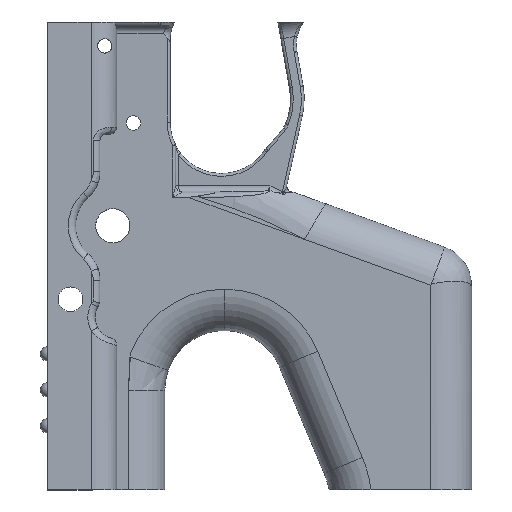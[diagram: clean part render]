
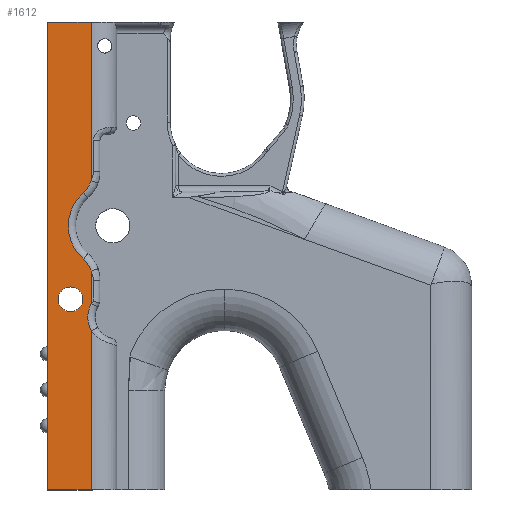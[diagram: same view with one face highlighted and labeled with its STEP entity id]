
A CAD part, left-side view. The second image highlights one B-rep face of the part: STEP entity #1612.
In plain terms, the highlighted planar face has unit normal (-1, 0, 0).
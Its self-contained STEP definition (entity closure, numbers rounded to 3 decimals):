
#29 = ORIENTED_EDGE ( 'NONE', *, *, #5917, .T. ) ;
#49 = ORIENTED_EDGE ( 'NONE', *, *, #7983, .F. ) ;
#68 = VERTEX_POINT ( 'NONE', #8819 ) ;
#126 = CARTESIAN_POINT ( 'NONE',  ( 4.253, 39.359, 4.07 ) ) ;
#310 = CARTESIAN_POINT ( 'NONE',  ( 4.253, 33.602, -8.151 ) ) ;
#328 = ORIENTED_EDGE ( 'NONE', *, *, #7733, .F. ) ;
#339 = EDGE_CURVE ( 'NONE', #5930, #7018, #5388, .T. ) ;
#431 = EDGE_CURVE ( 'NONE', #11280, #6899, #5611, .T. ) ;
#524 = ORIENTED_EDGE ( 'NONE', *, *, #3425, .F. ) ;
#691 = AXIS2_PLACEMENT_3D ( 'NONE', #8470, #8398, #8358 ) ;
#1302 = EDGE_LOOP ( 'NONE', ( #49, #524 ) ) ;
#1612 = ADVANCED_FACE ( 'NONE', ( #8592, #8515 ), #9590, .T. ) ;
#1860 = VERTEX_POINT ( 'NONE', #7393 ) ;
#1989 = EDGE_CURVE ( 'NONE', #10378, #4350, #9671, .T. ) ;
#2120 = EDGE_LOOP ( 'NONE', ( #10586, #9983, #5983, #11621, #10898, #5056, #29, #11926, #9533, #328 ) ) ;
#2543 = CARTESIAN_POINT ( 'NONE',  ( 4.253, 33.602, -52.337 ) ) ;
#2714 = EDGE_CURVE ( 'NONE', #4350, #5930, #12246, .T. ) ;
#2930 = CARTESIAN_POINT ( 'NONE',  ( 4.253, 39.359, 0.641 ) ) ;
#3131 = CARTESIAN_POINT ( 'NONE',  ( 4.253, 45.721, -52.337 ) ) ;
#3237 = LINE ( 'NONE', #7360, #3402 ) ;
#3402 = VECTOR ( 'NONE', #7688, 1000. ) ;
#3425 = EDGE_CURVE ( 'NONE', #6304, #6214, #4890, .T. ) ;
#3901 = DIRECTION ( 'NONE',  ( 0., 0., 1. ) ) ;
#3908 = VERTEX_POINT ( 'NONE', #3131 ) ;
#3967 = AXIS2_PLACEMENT_3D ( 'NONE', #4421, #3987, #4104 ) ;
#3987 = DIRECTION ( 'NONE',  ( 1., 0., 0. ) ) ;
#4104 = DIRECTION ( 'NONE',  ( 0., 0., 1. ) ) ;
#4350 = VERTEX_POINT ( 'NONE', #310 ) ;
#4421 = CARTESIAN_POINT ( 'NONE',  ( 4.253, 26.544, -4.363 ) ) ;
#4700 = DIRECTION ( 'NONE',  ( 0., 0., 1. ) ) ;
#4721 = CARTESIAN_POINT ( 'NONE',  ( 4.253, 33.602, 8.466 ) ) ;
#4752 = DIRECTION ( 'NONE',  ( 1., 0., 0. ) ) ;
#4765 = CARTESIAN_POINT ( 'NONE',  ( 4.253, 27.586, 21.037 ) ) ;
#4802 = CARTESIAN_POINT ( 'NONE',  ( 4.253, 35.831, 30.248 ) ) ;
#4890 = CIRCLE ( 'NONE', #691, 3.429 ) ;
#5056 = ORIENTED_EDGE ( 'NONE', *, *, #431, .T. ) ;
#5057 = AXIS2_PLACEMENT_3D ( 'NONE', #11637, #11622, #11606 ) ;
#5104 = DIRECTION ( 'NONE',  ( 0., 0., 1. ) ) ;
#5123 = EDGE_CURVE ( 'NONE', #7018, #12209, #7668, .T. ) ;
#5266 = CARTESIAN_POINT ( 'NONE',  ( 4.253, 41.167, 5.866 ) ) ;
#5302 = DIRECTION ( 'NONE',  ( -1., 0., 0. ) ) ;
#5388 = LINE ( 'NONE', #9391, #5407 ) ;
#5407 = VECTOR ( 'NONE', #9187, 1000. ) ;
#5438 = EDGE_CURVE ( 'NONE', #12209, #11280, #6070, .T. ) ;
#5611 = CIRCLE ( 'NONE', #5057, 8. ) ;
#5917 = EDGE_CURVE ( 'NONE', #6899, #68, #3237, .T. ) ;
#5930 = VERTEX_POINT ( 'NONE', #7248 ) ;
#5983 = ORIENTED_EDGE ( 'NONE', *, *, #339, .T. ) ;
#6025 = DIRECTION ( 'NONE',  ( 0., 0., 1. ) ) ;
#6070 = CIRCLE ( 'NONE', #11005, 12.362 ) ;
#6175 = AXIS2_PLACEMENT_3D ( 'NONE', #5266, #5302, #5104 ) ;
#6214 = VERTEX_POINT ( 'NONE', #126 ) ;
#6304 = VERTEX_POINT ( 'NONE', #10515 ) ;
#6432 = CARTESIAN_POINT ( 'NONE',  ( 4.253, 33.602, 141.062 ) ) ;
#6451 = CARTESIAN_POINT ( 'NONE',  ( 4.253, 45.721, 162.566 ) ) ;
#6594 = VECTOR ( 'NONE', #6025, 1000. ) ;
#6693 = EDGE_CURVE ( 'NONE', #68, #1860, #9528, .T. ) ;
#6883 = LINE ( 'NONE', #6451, #6594 ) ;
#6899 = VERTEX_POINT ( 'NONE', #11404 ) ;
#7006 = EDGE_CURVE ( 'NONE', #3908, #1860, #6883, .T. ) ;
#7018 = VERTEX_POINT ( 'NONE', #4721 ) ;
#7184 = DIRECTION ( 'NONE',  ( 0., 0., 1. ) ) ;
#7248 = CARTESIAN_POINT ( 'NONE',  ( 4.253, 33.602, -0.574 ) ) ;
#7360 = CARTESIAN_POINT ( 'NONE',  ( 4.253, 33.602, 141.062 ) ) ;
#7393 = CARTESIAN_POINT ( 'NONE',  ( 4.253, 45.721, 77.663 ) ) ;
#7534 = CARTESIAN_POINT ( 'NONE',  ( 4.253, 35.831, 11.827 ) ) ;
#7668 = CIRCLE ( 'NONE', #6175, 8. ) ;
#7688 = DIRECTION ( 'NONE',  ( 0., 0., 1. ) ) ;
#7733 = EDGE_CURVE ( 'NONE', #10378, #3908, #11584, .T. ) ;
#7983 = EDGE_CURVE ( 'NONE', #6214, #6304, #10690, .T. ) ;
#8259 = DIRECTION ( 'NONE',  ( 0., 1., 0. ) ) ;
#8270 = CARTESIAN_POINT ( 'NONE',  ( 4.253, 33.602, 77.663 ) ) ;
#8358 = DIRECTION ( 'NONE',  ( 0., 0., 1. ) ) ;
#8398 = DIRECTION ( 'NONE',  ( -1., 0., 0. ) ) ;
#8470 = CARTESIAN_POINT ( 'NONE',  ( 4.253, 39.359, 0.641 ) ) ;
#8515 = FACE_BOUND ( 'NONE', #1302, .T. ) ;
#8592 = FACE_OUTER_BOUND ( 'NONE', #2120, .T. ) ;
#8655 = CARTESIAN_POINT ( 'NONE',  ( 4.253, 33.602, -52.337 ) ) ;
#8819 = CARTESIAN_POINT ( 'NONE',  ( 4.253, 33.602, 77.663 ) ) ;
#9187 = DIRECTION ( 'NONE',  ( 0., 0., 1. ) ) ;
#9391 = CARTESIAN_POINT ( 'NONE',  ( 4.253, 33.602, 141.062 ) ) ;
#9400 = VECTOR ( 'NONE', #8259, 1000. ) ;
#9492 = AXIS2_PLACEMENT_3D ( 'NONE', #2930, #9553, #3901 ) ;
#9528 = LINE ( 'NONE', #8270, #9400 ) ;
#9533 = ORIENTED_EDGE ( 'NONE', *, *, #7006, .F. ) ;
#9553 = DIRECTION ( 'NONE',  ( -1., 0., 0. ) ) ;
#9585 = VECTOR ( 'NONE', #7184, 1000. ) ;
#9590 = PLANE ( 'NONE',  #11950 ) ;
#9671 = LINE ( 'NONE', #6432, #9585 ) ;
#9885 = CARTESIAN_POINT ( 'NONE',  ( 4.253, 33.602, 141.062 ) ) ;
#9926 = DIRECTION ( 'NONE',  ( -1., 0., 0. ) ) ;
#9983 = ORIENTED_EDGE ( 'NONE', *, *, #2714, .T. ) ;
#10008 = DIRECTION ( 'NONE',  ( 0., 0., 1. ) ) ;
#10084 = VECTOR ( 'NONE', #12009, 1000. ) ;
#10378 = VERTEX_POINT ( 'NONE', #8655 ) ;
#10515 = CARTESIAN_POINT ( 'NONE',  ( 4.253, 39.359, -2.788 ) ) ;
#10586 = ORIENTED_EDGE ( 'NONE', *, *, #1989, .T. ) ;
#10690 = CIRCLE ( 'NONE', #9492, 3.429 ) ;
#10898 = ORIENTED_EDGE ( 'NONE', *, *, #5438, .T. ) ;
#11005 = AXIS2_PLACEMENT_3D ( 'NONE', #4765, #4752, #4700 ) ;
#11280 = VERTEX_POINT ( 'NONE', #4802 ) ;
#11404 = CARTESIAN_POINT ( 'NONE',  ( 4.253, 33.602, 33.608 ) ) ;
#11584 = LINE ( 'NONE', #2543, #10084 ) ;
#11606 = DIRECTION ( 'NONE',  ( 0., 0., 1. ) ) ;
#11621 = ORIENTED_EDGE ( 'NONE', *, *, #5123, .T. ) ;
#11622 = DIRECTION ( 'NONE',  ( -1., 0., 0. ) ) ;
#11637 = CARTESIAN_POINT ( 'NONE',  ( 4.253, 41.167, 36.209 ) ) ;
#11926 = ORIENTED_EDGE ( 'NONE', *, *, #6693, .T. ) ;
#11950 = AXIS2_PLACEMENT_3D ( 'NONE', #9885, #9926, #10008 ) ;
#12009 = DIRECTION ( 'NONE',  ( 0., 1., 0. ) ) ;
#12209 = VERTEX_POINT ( 'NONE', #7534 ) ;
#12246 = CIRCLE ( 'NONE', #3967, 8.01 ) ;
